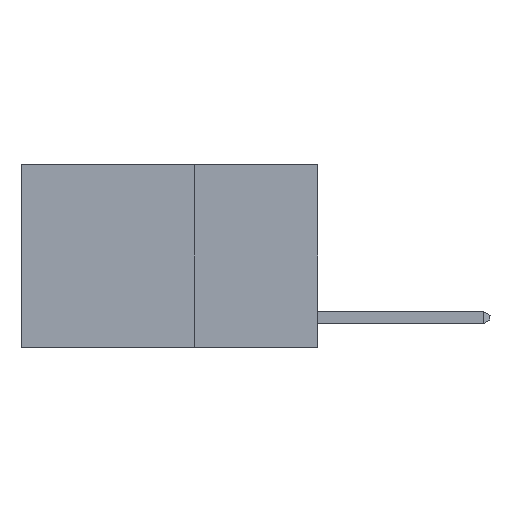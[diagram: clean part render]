
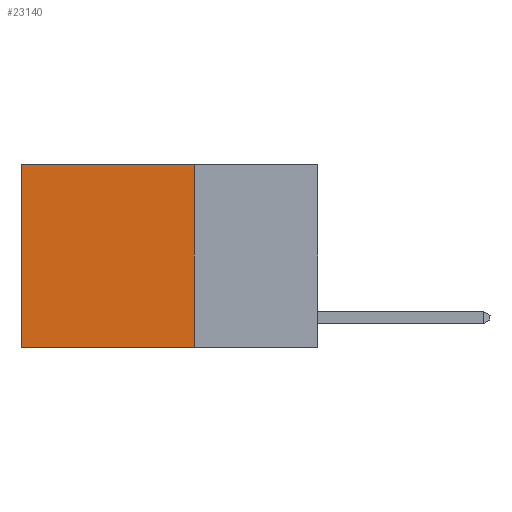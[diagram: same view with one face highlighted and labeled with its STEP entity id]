
A CAD part, left-side view. The second image highlights one B-rep face of the part: STEP entity #23140.
In plain terms, the highlighted planar face has unit normal (-1, 0, 0).
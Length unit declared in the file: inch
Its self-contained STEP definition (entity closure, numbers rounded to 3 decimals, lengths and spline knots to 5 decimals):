
#751 = VECTOR ( 'NONE', #15667, 39.37008 ) ;
#983 = LINE ( 'NONE', #23276, #5341 ) ;
#1144 = EDGE_CURVE ( 'NONE', #4958, #23286, #983, .T. ) ;
#1661 = LINE ( 'NONE', #18344, #5392 ) ;
#1873 = ORIENTED_EDGE ( 'NONE', *, *, #17391, .F. ) ;
#2270 = ORIENTED_EDGE ( 'NONE', *, *, #26273, .T. ) ;
#2819 = LINE ( 'NONE', #23982, #751 ) ;
#3232 = CARTESIAN_POINT ( 'NONE',  ( 0.2625, 0.25, -0.37 ) ) ;
#3458 = DIRECTION ( 'NONE',  ( 1., 0., 0. ) ) ;
#3669 = EDGE_CURVE ( 'NONE', #16905, #26962, #24284, .T. ) ;
#4020 = FACE_OUTER_BOUND ( 'NONE', #15593, .T. ) ;
#4040 = AXIS2_PLACEMENT_3D ( 'NONE', #22193, #3458, #16198 ) ;
#4958 = VERTEX_POINT ( 'NONE', #24021 ) ;
#5166 = CARTESIAN_POINT ( 'NONE',  ( 0.2625, 0.25, 0. ) ) ;
#5341 = VECTOR ( 'NONE', #17529, 39.37008 ) ;
#5392 = VECTOR ( 'NONE', #8091, 39.37008 ) ;
#8091 = DIRECTION ( 'NONE',  ( 0., 1., 0. ) ) ;
#13140 = CARTESIAN_POINT ( 'NONE',  ( 0.2625, 0.25, 0. ) ) ;
#13882 = PLANE ( 'NONE',  #4040 ) ;
#14813 = VECTOR ( 'NONE', #21980, 39.37008 ) ;
#15593 = EDGE_LOOP ( 'NONE', ( #16387, #1873, #18358, #2270 ) ) ;
#15667 = DIRECTION ( 'NONE',  ( 0., 1., 0. ) ) ;
#16198 = DIRECTION ( 'NONE',  ( 0., 0., -1. ) ) ;
#16387 = ORIENTED_EDGE ( 'NONE', *, *, #1144, .T. ) ;
#16905 = VERTEX_POINT ( 'NONE', #13140 ) ;
#17000 = CARTESIAN_POINT ( 'NONE',  ( 0.2625, 0.6, -0.37 ) ) ;
#17391 = EDGE_CURVE ( 'NONE', #26962, #23286, #2819, .T. ) ;
#17529 = DIRECTION ( 'NONE',  ( 0., 0., -1. ) ) ;
#18344 = CARTESIAN_POINT ( 'NONE',  ( 0.2625, 0.25, 0. ) ) ;
#18358 = ORIENTED_EDGE ( 'NONE', *, *, #3669, .F. ) ;
#21980 = DIRECTION ( 'NONE',  ( 0., 0., -1. ) ) ;
#22193 = CARTESIAN_POINT ( 'NONE',  ( 0.2625, 0.25, 0. ) ) ;
#23140 = ADVANCED_FACE ( 'NONE', ( #4020 ), #13882, .F. ) ;
#23276 = CARTESIAN_POINT ( 'NONE',  ( 0.2625, 0.6, 0. ) ) ;
#23286 = VERTEX_POINT ( 'NONE', #17000 ) ;
#23982 = CARTESIAN_POINT ( 'NONE',  ( 0.2625, 0.25, -0.37 ) ) ;
#24021 = CARTESIAN_POINT ( 'NONE',  ( 0.2625, 0.6, 0. ) ) ;
#24284 = LINE ( 'NONE', #5166, #14813 ) ;
#26273 = EDGE_CURVE ( 'NONE', #16905, #4958, #1661, .T. ) ;
#26962 = VERTEX_POINT ( 'NONE', #3232 ) ;
